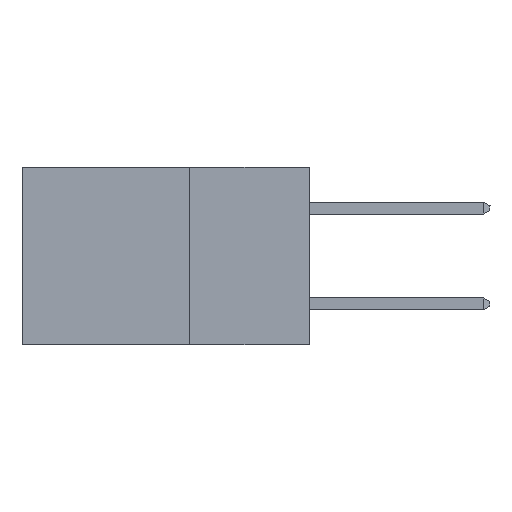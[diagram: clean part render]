
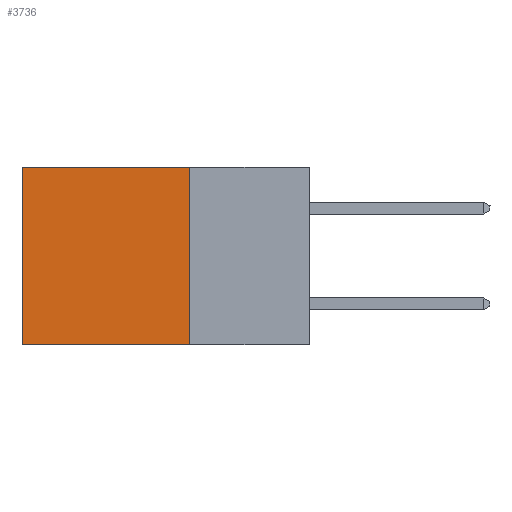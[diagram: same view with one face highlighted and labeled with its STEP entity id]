
A CAD part, left-side view. The second image highlights one B-rep face of the part: STEP entity #3736.
In plain terms, the highlighted planar face has unit normal (-1, 0, 0).
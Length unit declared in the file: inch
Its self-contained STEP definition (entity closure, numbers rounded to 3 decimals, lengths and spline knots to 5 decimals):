
#226 = VERTEX_POINT ( 'NONE', #1415 ) ;
#495 = LINE ( 'NONE', #10088, #6039 ) ;
#1059 = VECTOR ( 'NONE', #8296, 39.37008 ) ;
#1304 = CARTESIAN_POINT ( 'NONE',  ( 0.2875, 0.25, -0.37 ) ) ;
#1415 = CARTESIAN_POINT ( 'NONE',  ( 0.2875, 0.6, 0. ) ) ;
#1577 = FACE_OUTER_BOUND ( 'NONE', #2998, .T. ) ;
#2155 = VECTOR ( 'NONE', #2697, 39.37008 ) ;
#2697 = DIRECTION ( 'NONE',  ( 0., 1., 0. ) ) ;
#2998 = EDGE_LOOP ( 'NONE', ( #10848, #10395, #6718, #11855 ) ) ;
#3736 = ADVANCED_FACE ( 'NONE', ( #1577 ), #9036, .F. ) ;
#4538 = EDGE_CURVE ( 'NONE', #8698, #7696, #11312, .T. ) ;
#4675 = DIRECTION ( 'NONE',  ( 0., 0., -1. ) ) ;
#4971 = DIRECTION ( 'NONE',  ( 0., 0., -1. ) ) ;
#6039 = VECTOR ( 'NONE', #4675, 39.37008 ) ;
#6718 = ORIENTED_EDGE ( 'NONE', *, *, #13452, .F. ) ;
#7696 = VERTEX_POINT ( 'NONE', #9388 ) ;
#7909 = AXIS2_PLACEMENT_3D ( 'NONE', #13586, #9174, #4971 ) ;
#8177 = CARTESIAN_POINT ( 'NONE',  ( 0.2875, 0.25, 0. ) ) ;
#8296 = DIRECTION ( 'NONE',  ( 0., 0., -1. ) ) ;
#8698 = VERTEX_POINT ( 'NONE', #1304 ) ;
#9036 = PLANE ( 'NONE',  #7909 ) ;
#9174 = DIRECTION ( 'NONE',  ( 1., 0., 0. ) ) ;
#9349 = LINE ( 'NONE', #13494, #1059 ) ;
#9388 = CARTESIAN_POINT ( 'NONE',  ( 0.2875, 0.6, -0.37 ) ) ;
#9817 = EDGE_CURVE ( 'NONE', #12463, #226, #12392, .T. ) ;
#10088 = CARTESIAN_POINT ( 'NONE',  ( 0.2875, 0.25, 0. ) ) ;
#10395 = ORIENTED_EDGE ( 'NONE', *, *, #4538, .F. ) ;
#10848 = ORIENTED_EDGE ( 'NONE', *, *, #12881, .T. ) ;
#11102 = DIRECTION ( 'NONE',  ( 0., 1., 0. ) ) ;
#11175 = CARTESIAN_POINT ( 'NONE',  ( 0.2875, 0.25, -0.37 ) ) ;
#11312 = LINE ( 'NONE', #11175, #11567 ) ;
#11567 = VECTOR ( 'NONE', #11102, 39.37008 ) ;
#11855 = ORIENTED_EDGE ( 'NONE', *, *, #9817, .T. ) ;
#12328 = CARTESIAN_POINT ( 'NONE',  ( 0.2875, 0.25, 0. ) ) ;
#12392 = LINE ( 'NONE', #12328, #2155 ) ;
#12463 = VERTEX_POINT ( 'NONE', #8177 ) ;
#12881 = EDGE_CURVE ( 'NONE', #226, #7696, #9349, .T. ) ;
#13452 = EDGE_CURVE ( 'NONE', #12463, #8698, #495, .T. ) ;
#13494 = CARTESIAN_POINT ( 'NONE',  ( 0.2875, 0.6, 0. ) ) ;
#13586 = CARTESIAN_POINT ( 'NONE',  ( 0.2875, 0.25, 0. ) ) ;
